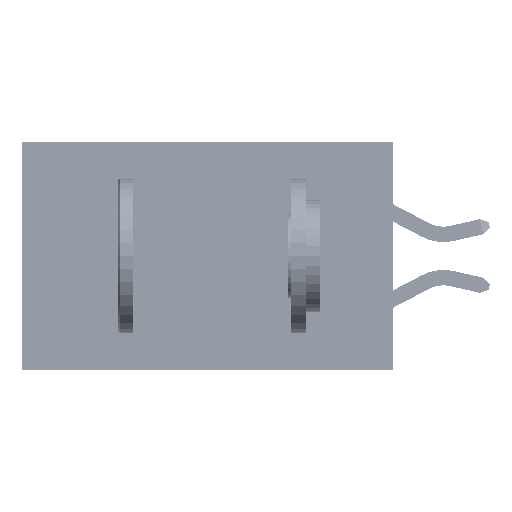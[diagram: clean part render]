
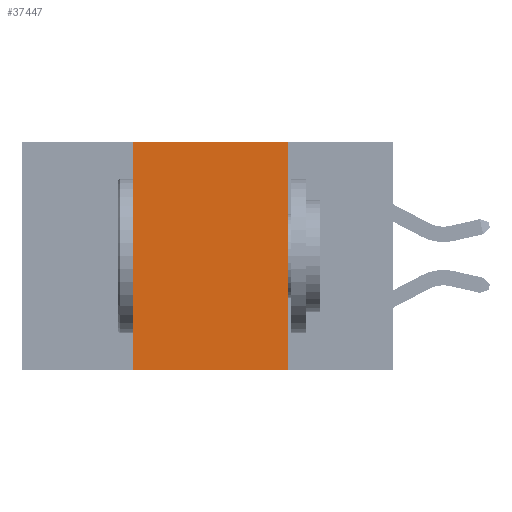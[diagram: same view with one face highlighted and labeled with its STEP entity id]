
A CAD part, left-side view. The second image highlights one B-rep face of the part: STEP entity #37447.
In plain terms, the highlighted planar face has unit normal (-1, 0, 0).
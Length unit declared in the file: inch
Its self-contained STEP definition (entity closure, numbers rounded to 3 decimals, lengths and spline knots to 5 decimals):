
#1260 = LINE ( 'NONE', #15581, #37176 ) ;
#3839 = CARTESIAN_POINT ( 'NONE',  ( 0., 0.6, 0. ) ) ;
#5955 = VERTEX_POINT ( 'NONE', #29595 ) ;
#7349 = DIRECTION ( 'NONE',  ( 1., 0., 0. ) ) ;
#9756 = FACE_OUTER_BOUND ( 'NONE', #11314, .T. ) ;
#9789 = EDGE_CURVE ( 'NONE', #36292, #37590, #1260, .T. ) ;
#10270 = EDGE_CURVE ( 'NONE', #5955, #29632, #27928, .T. ) ;
#11144 = DIRECTION ( 'NONE',  ( 0., -1., 0. ) ) ;
#11286 = CARTESIAN_POINT ( 'NONE',  ( 0., 0.17, 0. ) ) ;
#11314 = EDGE_LOOP ( 'NONE', ( #17245, #40179, #35732, #19119 ) ) ;
#13631 = EDGE_CURVE ( 'NONE', #5955, #36292, #43476, .T. ) ;
#13837 = VECTOR ( 'NONE', #31684, 39.37008 ) ;
#15581 = CARTESIAN_POINT ( 'NONE',  ( 0., 0.6, 0. ) ) ;
#17245 = ORIENTED_EDGE ( 'NONE', *, *, #19931, .F. ) ;
#19087 = DIRECTION ( 'NONE',  ( 0., -1., 0. ) ) ;
#19119 = ORIENTED_EDGE ( 'NONE', *, *, #10270, .T. ) ;
#19931 = EDGE_CURVE ( 'NONE', #37590, #29632, #23040, .T. ) ;
#21030 = CARTESIAN_POINT ( 'NONE',  ( 0., 0.17, 0. ) ) ;
#23040 = LINE ( 'NONE', #21030, #13837 ) ;
#24659 = PLANE ( 'NONE',  #40502 ) ;
#26484 = CARTESIAN_POINT ( 'NONE',  ( 0., 0.42, 0. ) ) ;
#27928 = LINE ( 'NONE', #42318, #36036 ) ;
#29595 = CARTESIAN_POINT ( 'NONE',  ( 0., 0.42, -0.37 ) ) ;
#29632 = VERTEX_POINT ( 'NONE', #41355 ) ;
#31671 = DIRECTION ( 'NONE',  ( 0., 0., -1. ) ) ;
#31684 = DIRECTION ( 'NONE',  ( 0., 0., -1. ) ) ;
#35096 = CARTESIAN_POINT ( 'NONE',  ( 0., 0.42, 0. ) ) ;
#35732 = ORIENTED_EDGE ( 'NONE', *, *, #13631, .F. ) ;
#36036 = VECTOR ( 'NONE', #11144, 39.37008 ) ;
#36292 = VERTEX_POINT ( 'NONE', #35096 ) ;
#36828 = DIRECTION ( 'NONE',  ( 0., 0., 1. ) ) ;
#37176 = VECTOR ( 'NONE', #19087, 39.37008 ) ;
#37447 = ADVANCED_FACE ( 'NONE', ( #9756 ), #24659, .F. ) ;
#37590 = VERTEX_POINT ( 'NONE', #11286 ) ;
#40179 = ORIENTED_EDGE ( 'NONE', *, *, #9789, .F. ) ;
#40502 = AXIS2_PLACEMENT_3D ( 'NONE', #3839, #7349, #31671 ) ;
#41355 = CARTESIAN_POINT ( 'NONE',  ( 0., 0.17, -0.37 ) ) ;
#42318 = CARTESIAN_POINT ( 'NONE',  ( 0., 0.6, -0.37 ) ) ;
#43476 = LINE ( 'NONE', #26484, #44584 ) ;
#44584 = VECTOR ( 'NONE', #36828, 39.37008 ) ;
